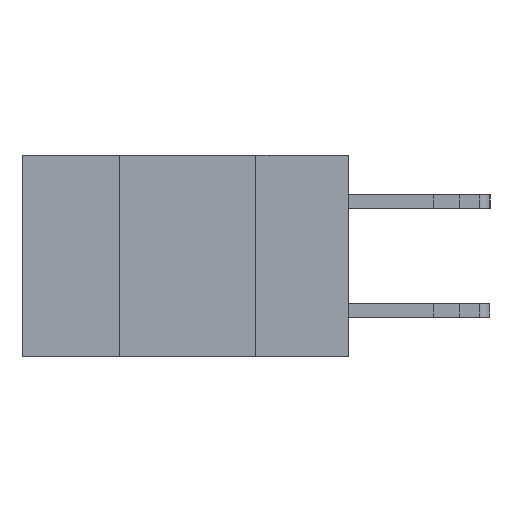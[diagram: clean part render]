
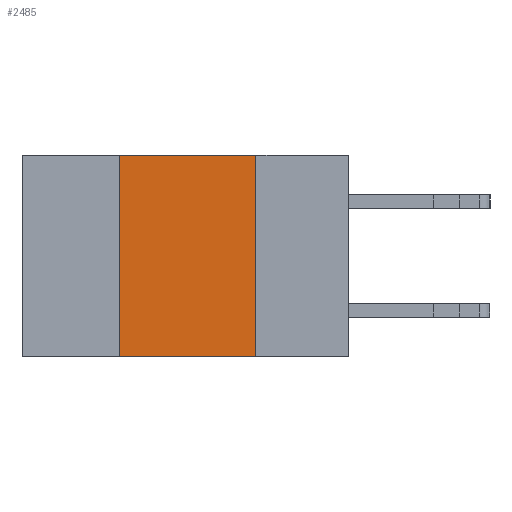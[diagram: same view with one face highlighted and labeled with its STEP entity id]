
A CAD part, left-side view. The second image highlights one B-rep face of the part: STEP entity #2485.
In plain terms, the highlighted planar face has unit normal (-1, 0, 0).
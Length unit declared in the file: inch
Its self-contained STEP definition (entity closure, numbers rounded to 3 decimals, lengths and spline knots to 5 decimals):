
#252 = PLANE ( 'NONE',  #12032 ) ;
#1874 = VERTEX_POINT ( 'NONE', #16069 ) ;
#2006 = DIRECTION ( 'NONE',  ( 0., 0., -1. ) ) ;
#2306 = LINE ( 'NONE', #3905, #15510 ) ;
#2345 = DIRECTION ( 'NONE',  ( 1., 0., 0. ) ) ;
#2461 = DIRECTION ( 'NONE',  ( 0., 0., -1. ) ) ;
#2485 = ADVANCED_FACE ( 'NONE', ( #3139 ), #252, .F. ) ;
#3139 = FACE_OUTER_BOUND ( 'NONE', #3301, .T. ) ;
#3281 = LINE ( 'NONE', #8836, #16466 ) ;
#3301 = EDGE_LOOP ( 'NONE', ( #8498, #8280, #7839, #5859 ) ) ;
#3428 = VECTOR ( 'NONE', #11042, 39.37008 ) ;
#3484 = EDGE_CURVE ( 'NONE', #8488, #1874, #7714, .T. ) ;
#3905 = CARTESIAN_POINT ( 'NONE',  ( 0., 0.42, 0. ) ) ;
#4027 = VERTEX_POINT ( 'NONE', #8687 ) ;
#4307 = VECTOR ( 'NONE', #5392, 39.37008 ) ;
#4945 = CARTESIAN_POINT ( 'NONE',  ( 0., 0.6, 0. ) ) ;
#5216 = EDGE_CURVE ( 'NONE', #4027, #13743, #14073, .T. ) ;
#5392 = DIRECTION ( 'NONE',  ( 0., -1., 0. ) ) ;
#5859 = ORIENTED_EDGE ( 'NONE', *, *, #5216, .T. ) ;
#7714 = LINE ( 'NONE', #4945, #4307 ) ;
#7839 = ORIENTED_EDGE ( 'NONE', *, *, #16140, .F. ) ;
#8280 = ORIENTED_EDGE ( 'NONE', *, *, #3484, .F. ) ;
#8488 = VERTEX_POINT ( 'NONE', #10424 ) ;
#8498 = ORIENTED_EDGE ( 'NONE', *, *, #10490, .F. ) ;
#8687 = CARTESIAN_POINT ( 'NONE',  ( 0., 0.42, -0.37 ) ) ;
#8836 = CARTESIAN_POINT ( 'NONE',  ( 0., 0.17, 0. ) ) ;
#10424 = CARTESIAN_POINT ( 'NONE',  ( 0., 0.42, 0. ) ) ;
#10490 = EDGE_CURVE ( 'NONE', #1874, #13743, #3281, .T. ) ;
#11042 = DIRECTION ( 'NONE',  ( 0., -1., 0. ) ) ;
#11683 = DIRECTION ( 'NONE',  ( 0., 0., 1. ) ) ;
#11750 = CARTESIAN_POINT ( 'NONE',  ( 0., 0.17, -0.37 ) ) ;
#12032 = AXIS2_PLACEMENT_3D ( 'NONE', #14669, #2345, #2006 ) ;
#13743 = VERTEX_POINT ( 'NONE', #11750 ) ;
#14073 = LINE ( 'NONE', #14908, #3428 ) ;
#14669 = CARTESIAN_POINT ( 'NONE',  ( 0., 0.6, 0. ) ) ;
#14908 = CARTESIAN_POINT ( 'NONE',  ( 0., 0.6, -0.37 ) ) ;
#15510 = VECTOR ( 'NONE', #11683, 39.37008 ) ;
#16069 = CARTESIAN_POINT ( 'NONE',  ( 0., 0.17, 0. ) ) ;
#16140 = EDGE_CURVE ( 'NONE', #4027, #8488, #2306, .T. ) ;
#16466 = VECTOR ( 'NONE', #2461, 39.37008 ) ;
